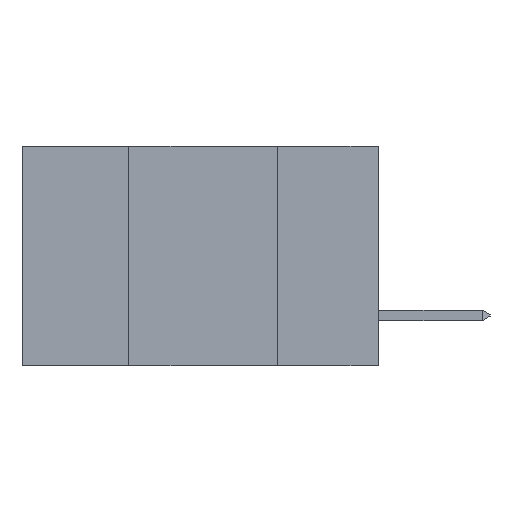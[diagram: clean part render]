
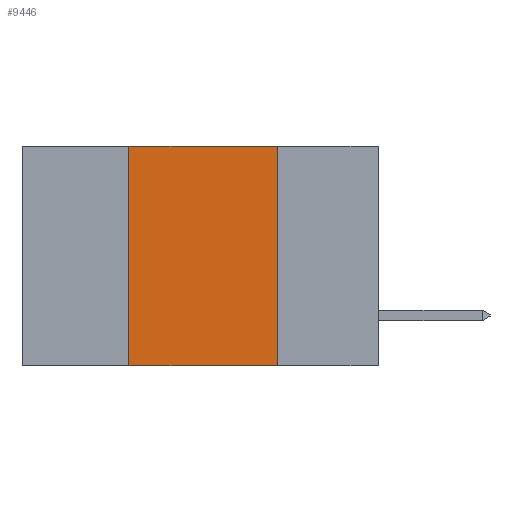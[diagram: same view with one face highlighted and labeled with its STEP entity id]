
A CAD part, left-side view. The second image highlights one B-rep face of the part: STEP entity #9446.
In plain terms, the highlighted planar face has unit normal (-1, 0, 0).
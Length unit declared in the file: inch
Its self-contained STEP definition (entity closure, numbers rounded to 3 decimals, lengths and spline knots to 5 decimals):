
#1 = LINE ( 'NONE', #4491, #2856 ) ;
#274 = CARTESIAN_POINT ( 'NONE',  ( 0., 0.17, 0. ) ) ;
#815 = ORIENTED_EDGE ( 'NONE', *, *, #13739, .F. ) ;
#939 = DIRECTION ( 'NONE',  ( 0., -1., 0. ) ) ;
#1159 = CARTESIAN_POINT ( 'NONE',  ( 0., 0.42, -0.37 ) ) ;
#1178 = EDGE_CURVE ( 'NONE', #2057, #11142, #2179, .T. ) ;
#2057 = VERTEX_POINT ( 'NONE', #274 ) ;
#2179 = LINE ( 'NONE', #2239, #4535 ) ;
#2239 = CARTESIAN_POINT ( 'NONE',  ( 0., 0.17, 0. ) ) ;
#2279 = LINE ( 'NONE', #9806, #5013 ) ;
#2856 = VECTOR ( 'NONE', #939, 39.37008 ) ;
#3661 = AXIS2_PLACEMENT_3D ( 'NONE', #5537, #14589, #7825 ) ;
#3800 = DIRECTION ( 'NONE',  ( 0., 0., -1. ) ) ;
#4491 = CARTESIAN_POINT ( 'NONE',  ( 0., 0.6, -0.37 ) ) ;
#4535 = VECTOR ( 'NONE', #3800, 39.37008 ) ;
#5013 = VECTOR ( 'NONE', #10521, 39.37008 ) ;
#5536 = ORIENTED_EDGE ( 'NONE', *, *, #12984, .T. ) ;
#5537 = CARTESIAN_POINT ( 'NONE',  ( 0., 0.6, 0. ) ) ;
#6471 = VERTEX_POINT ( 'NONE', #1159 ) ;
#6847 = ORIENTED_EDGE ( 'NONE', *, *, #1178, .F. ) ;
#7316 = EDGE_CURVE ( 'NONE', #8686, #2057, #10495, .T. ) ;
#7464 = VECTOR ( 'NONE', #10919, 39.37008 ) ;
#7753 = ORIENTED_EDGE ( 'NONE', *, *, #7316, .F. ) ;
#7825 = DIRECTION ( 'NONE',  ( 0., 0., -1. ) ) ;
#8686 = VERTEX_POINT ( 'NONE', #11143 ) ;
#9446 = ADVANCED_FACE ( 'NONE', ( #10628 ), #13462, .F. ) ;
#9806 = CARTESIAN_POINT ( 'NONE',  ( 0., 0.42, 0. ) ) ;
#10305 = CARTESIAN_POINT ( 'NONE',  ( 0., 0.6, 0. ) ) ;
#10495 = LINE ( 'NONE', #10305, #7464 ) ;
#10521 = DIRECTION ( 'NONE',  ( 0., 0., 1. ) ) ;
#10628 = FACE_OUTER_BOUND ( 'NONE', #12204, .T. ) ;
#10720 = CARTESIAN_POINT ( 'NONE',  ( 0., 0.17, -0.37 ) ) ;
#10919 = DIRECTION ( 'NONE',  ( 0., -1., 0. ) ) ;
#11142 = VERTEX_POINT ( 'NONE', #10720 ) ;
#11143 = CARTESIAN_POINT ( 'NONE',  ( 0., 0.42, 0. ) ) ;
#12204 = EDGE_LOOP ( 'NONE', ( #6847, #7753, #815, #5536 ) ) ;
#12984 = EDGE_CURVE ( 'NONE', #6471, #11142, #1, .T. ) ;
#13462 = PLANE ( 'NONE',  #3661 ) ;
#13739 = EDGE_CURVE ( 'NONE', #6471, #8686, #2279, .T. ) ;
#14589 = DIRECTION ( 'NONE',  ( 1., 0., 0. ) ) ;
